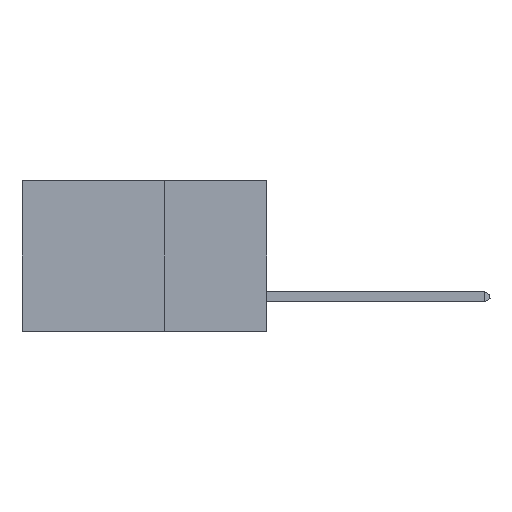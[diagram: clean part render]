
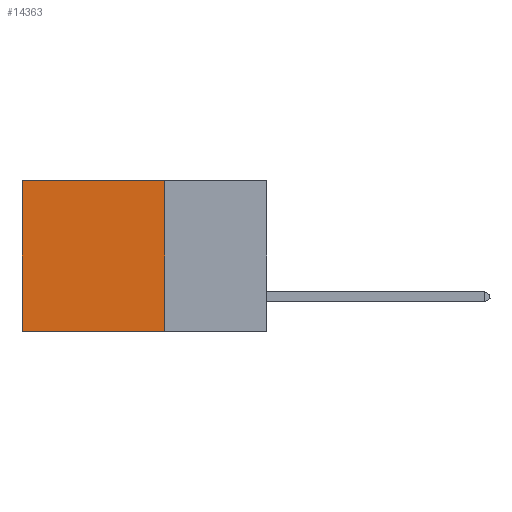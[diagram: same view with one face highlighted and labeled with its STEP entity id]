
A CAD part, left-side view. The second image highlights one B-rep face of the part: STEP entity #14363.
In plain terms, the highlighted planar face has unit normal (-1, 0, 0).
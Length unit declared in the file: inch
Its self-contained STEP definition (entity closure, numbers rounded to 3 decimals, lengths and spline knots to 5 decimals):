
#1372 = CARTESIAN_POINT ( 'NONE',  ( 0.2875, 0.25, -0.37 ) ) ;
#1864 = LINE ( 'NONE', #4450, #19598 ) ;
#2443 = DIRECTION ( 'NONE',  ( 0., 0., -1. ) ) ;
#3365 = CARTESIAN_POINT ( 'NONE',  ( 0.2875, 0.6, -0.37 ) ) ;
#3993 = CARTESIAN_POINT ( 'NONE',  ( 0.2875, 0.25, 0. ) ) ;
#4450 = CARTESIAN_POINT ( 'NONE',  ( 0.2875, 0.6, 0. ) ) ;
#4606 = EDGE_CURVE ( 'NONE', #5653, #13788, #16743, .T. ) ;
#5397 = ORIENTED_EDGE ( 'NONE', *, *, #15449, .T. ) ;
#5533 = CARTESIAN_POINT ( 'NONE',  ( 0.2875, 0.25, 0. ) ) ;
#5653 = VERTEX_POINT ( 'NONE', #6758 ) ;
#6758 = CARTESIAN_POINT ( 'NONE',  ( 0.2875, 0.25, 0. ) ) ;
#6918 = CARTESIAN_POINT ( 'NONE',  ( 0.2875, 0.25, -0.37 ) ) ;
#7021 = DIRECTION ( 'NONE',  ( 0., 1., 0. ) ) ;
#7216 = EDGE_LOOP ( 'NONE', ( #16868, #9885, #22009, #5397 ) ) ;
#7723 = PLANE ( 'NONE',  #11615 ) ;
#8234 = VECTOR ( 'NONE', #17929, 39.37008 ) ;
#9885 = ORIENTED_EDGE ( 'NONE', *, *, #22750, .F. ) ;
#11195 = DIRECTION ( 'NONE',  ( 1., 0., 0. ) ) ;
#11292 = EDGE_CURVE ( 'NONE', #17739, #18487, #1864, .T. ) ;
#11615 = AXIS2_PLACEMENT_3D ( 'NONE', #12920, #11195, #18434 ) ;
#12920 = CARTESIAN_POINT ( 'NONE',  ( 0.2875, 0.25, 0. ) ) ;
#13788 = VERTEX_POINT ( 'NONE', #6918 ) ;
#14363 = ADVANCED_FACE ( 'NONE', ( #22985 ), #7723, .F. ) ;
#15449 = EDGE_CURVE ( 'NONE', #5653, #17739, #22383, .T. ) ;
#15633 = VECTOR ( 'NONE', #2443, 39.37008 ) ;
#16743 = LINE ( 'NONE', #3993, #15633 ) ;
#16868 = ORIENTED_EDGE ( 'NONE', *, *, #11292, .T. ) ;
#17739 = VERTEX_POINT ( 'NONE', #19066 ) ;
#17929 = DIRECTION ( 'NONE',  ( 0., 1., 0. ) ) ;
#18405 = DIRECTION ( 'NONE',  ( 0., 0., -1. ) ) ;
#18434 = DIRECTION ( 'NONE',  ( 0., 0., -1. ) ) ;
#18487 = VERTEX_POINT ( 'NONE', #3365 ) ;
#19066 = CARTESIAN_POINT ( 'NONE',  ( 0.2875, 0.6, 0. ) ) ;
#19598 = VECTOR ( 'NONE', #18405, 39.37008 ) ;
#19643 = VECTOR ( 'NONE', #7021, 39.37008 ) ;
#20438 = LINE ( 'NONE', #1372, #19643 ) ;
#22009 = ORIENTED_EDGE ( 'NONE', *, *, #4606, .F. ) ;
#22383 = LINE ( 'NONE', #5533, #8234 ) ;
#22750 = EDGE_CURVE ( 'NONE', #13788, #18487, #20438, .T. ) ;
#22985 = FACE_OUTER_BOUND ( 'NONE', #7216, .T. ) ;
